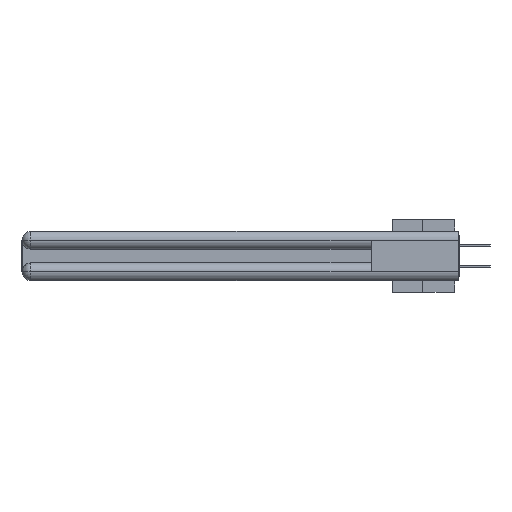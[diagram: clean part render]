
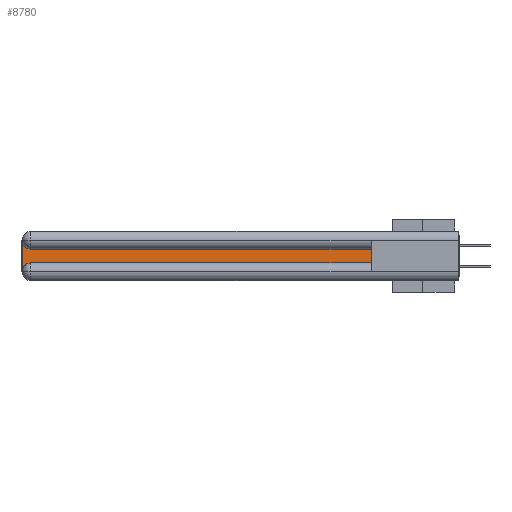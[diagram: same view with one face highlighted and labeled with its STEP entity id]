
A CAD part, left-side view. The second image highlights one B-rep face of the part: STEP entity #8780.
In plain terms, the highlighted planar face has unit normal (-1, 0, 0).
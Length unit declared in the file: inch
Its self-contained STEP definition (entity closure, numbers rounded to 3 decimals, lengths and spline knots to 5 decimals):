
#18 = CARTESIAN_POINT ( 'NONE',  ( 0.075, 0.6, -0.2175 ) ) ;
#1612 = VERTEX_POINT ( 'NONE', #18 ) ;
#1795 = VERTEX_POINT ( 'NONE', #37047 ) ;
#2431 = AXIS2_PLACEMENT_3D ( 'NONE', #20179, #16655, #16826 ) ;
#3066 = DIRECTION ( 'NONE',  ( 0., 0., -1. ) ) ;
#6121 = EDGE_CURVE ( 'NONE', #13625, #1612, #23771, .T. ) ;
#6129 = DIRECTION ( 'NONE',  ( 0., 1., 0. ) ) ;
#7691 = CIRCLE ( 'NONE', #25908, 0.06 ) ;
#8780 = ADVANCED_FACE ( 'NONE', ( #36867 ), #39306, .F. ) ;
#10238 = DIRECTION ( 'NONE',  ( 1., 0., 0. ) ) ;
#12766 = VECTOR ( 'NONE', #36562, 39.37008 ) ;
#13004 = VERTEX_POINT ( 'NONE', #40010 ) ;
#13118 = CARTESIAN_POINT ( 'NONE',  ( 0.075, 2.94, -0.2775 ) ) ;
#13272 = CARTESIAN_POINT ( 'NONE',  ( 0.075, 0.6, -0.1225 ) ) ;
#13625 = VERTEX_POINT ( 'NONE', #34850 ) ;
#13975 = VECTOR ( 'NONE', #6129, 39.37008 ) ;
#14454 = EDGE_CURVE ( 'NONE', #1795, #13625, #7691, .T. ) ;
#15222 = LINE ( 'NONE', #31675, #21528 ) ;
#15365 = EDGE_CURVE ( 'NONE', #39120, #1795, #15222, .T. ) ;
#16655 = DIRECTION ( 'NONE',  ( 1., 0., 0. ) ) ;
#16826 = DIRECTION ( 'NONE',  ( 0., 0., -1. ) ) ;
#16855 = ORIENTED_EDGE ( 'NONE', *, *, #6121, .T. ) ;
#16973 = CARTESIAN_POINT ( 'NONE',  ( 0.075, 0.6, -0.2175 ) ) ;
#18355 = DIRECTION ( 'NONE',  ( 0., 0., -1. ) ) ;
#19131 = LINE ( 'NONE', #16973, #32625 ) ;
#19148 = CARTESIAN_POINT ( 'NONE',  ( 0.075, 3., -0.0625 ) ) ;
#20179 = CARTESIAN_POINT ( 'NONE',  ( 0.075, 2.94, -0.0625 ) ) ;
#20297 = DIRECTION ( 'NONE',  ( 1., 0., 0. ) ) ;
#21528 = VECTOR ( 'NONE', #18355, 39.37008 ) ;
#21749 = ORIENTED_EDGE ( 'NONE', *, *, #14454, .T. ) ;
#22802 = LINE ( 'NONE', #13272, #13975 ) ;
#23150 = CARTESIAN_POINT ( 'NONE',  ( 0.075, 0.6, -0.2175 ) ) ;
#23771 = LINE ( 'NONE', #23150, #12766 ) ;
#23941 = DIRECTION ( 'NONE',  ( 0., 0., -1. ) ) ;
#24073 = CIRCLE ( 'NONE', #2431, 0.06 ) ;
#24716 = ORIENTED_EDGE ( 'NONE', *, *, #26226, .T. ) ;
#25908 = AXIS2_PLACEMENT_3D ( 'NONE', #13118, #10238, #3066 ) ;
#26226 = EDGE_CURVE ( 'NONE', #1612, #13004, #19131, .T. ) ;
#31191 = EDGE_LOOP ( 'NONE', ( #42354, #37634, #39338, #21749, #16855, #24716 ) ) ;
#31675 = CARTESIAN_POINT ( 'NONE',  ( 0.075, 3., -0.2175 ) ) ;
#32625 = VECTOR ( 'NONE', #41598, 39.37008 ) ;
#33726 = EDGE_CURVE ( 'NONE', #34047, #39120, #24073, .T. ) ;
#34047 = VERTEX_POINT ( 'NONE', #39143 ) ;
#34770 = AXIS2_PLACEMENT_3D ( 'NONE', #36235, #20297, #23941 ) ;
#34850 = CARTESIAN_POINT ( 'NONE',  ( 0.075, 2.94, -0.2175 ) ) ;
#36235 = CARTESIAN_POINT ( 'NONE',  ( 0.075, 3., -0.1225 ) ) ;
#36562 = DIRECTION ( 'NONE',  ( 0., -1., 0. ) ) ;
#36867 = FACE_OUTER_BOUND ( 'NONE', #31191, .T. ) ;
#37047 = CARTESIAN_POINT ( 'NONE',  ( 0.075, 3., -0.2775 ) ) ;
#37634 = ORIENTED_EDGE ( 'NONE', *, *, #33726, .T. ) ;
#39120 = VERTEX_POINT ( 'NONE', #19148 ) ;
#39143 = CARTESIAN_POINT ( 'NONE',  ( 0.075, 2.94, -0.1225 ) ) ;
#39306 = PLANE ( 'NONE',  #34770 ) ;
#39338 = ORIENTED_EDGE ( 'NONE', *, *, #15365, .T. ) ;
#40010 = CARTESIAN_POINT ( 'NONE',  ( 0.075, 0.6, -0.1225 ) ) ;
#40526 = EDGE_CURVE ( 'NONE', #13004, #34047, #22802, .T. ) ;
#41598 = DIRECTION ( 'NONE',  ( 0., 0., 1. ) ) ;
#42354 = ORIENTED_EDGE ( 'NONE', *, *, #40526, .T. ) ;
